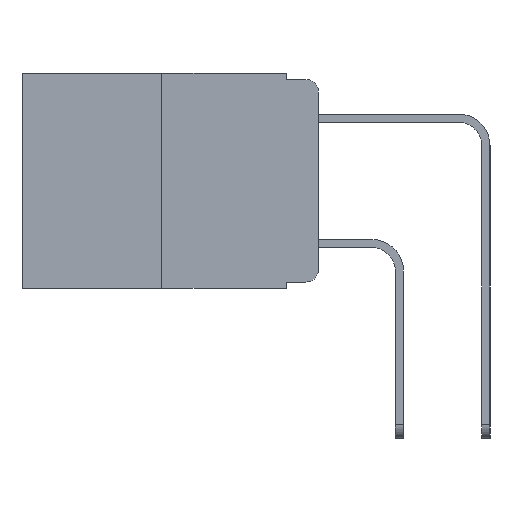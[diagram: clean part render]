
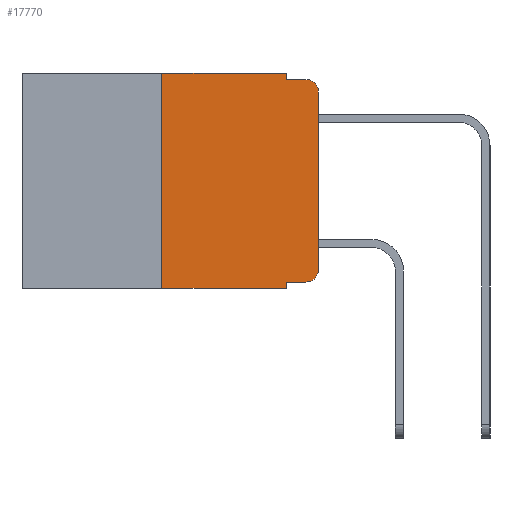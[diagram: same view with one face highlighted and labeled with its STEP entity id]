
A CAD part, left-side view. The second image highlights one B-rep face of the part: STEP entity #17770.
In plain terms, the highlighted planar face has unit normal (-1, 0, 0).
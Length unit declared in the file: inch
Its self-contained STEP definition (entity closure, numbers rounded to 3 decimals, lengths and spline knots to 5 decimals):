
#58 = VECTOR ( 'NONE', #22127, 39.37008 ) ;
#187 = DIRECTION ( 'NONE',  ( 0., 0., -1. ) ) ;
#230 = VERTEX_POINT ( 'NONE', #7218 ) ;
#246 = VERTEX_POINT ( 'NONE', #20464 ) ;
#477 = DIRECTION ( 'NONE',  ( 0., -1., 0. ) ) ;
#1325 = ORIENTED_EDGE ( 'NONE', *, *, #17352, .T. ) ;
#2344 = VERTEX_POINT ( 'NONE', #15406 ) ;
#2471 = VECTOR ( 'NONE', #20257, 39.37008 ) ;
#2782 = EDGE_LOOP ( 'NONE', ( #2958, #1325, #15148, #18935, #14340, #17602, #11539, #19645, #6774, #20719 ) ) ;
#2958 = ORIENTED_EDGE ( 'NONE', *, *, #18507, .T. ) ;
#3622 = CARTESIAN_POINT ( 'NONE',  ( 0., 0.25, 0. ) ) ;
#4239 = VERTEX_POINT ( 'NONE', #12228 ) ;
#4862 = CARTESIAN_POINT ( 'NONE',  ( 0., 0.051, 0. ) ) ;
#4883 = CARTESIAN_POINT ( 'NONE',  ( 0., 0.473, 0. ) ) ;
#5022 = LINE ( 'NONE', #14661, #21909 ) ;
#5245 = VERTEX_POINT ( 'NONE', #15235 ) ;
#5593 = EDGE_CURVE ( 'NONE', #4239, #2344, #10054, .T. ) ;
#6008 = VERTEX_POINT ( 'NONE', #19014 ) ;
#6492 = CARTESIAN_POINT ( 'NONE',  ( 0., 0.473, 0. ) ) ;
#6739 = EDGE_CURVE ( 'NONE', #15500, #4239, #17334, .T. ) ;
#6774 = ORIENTED_EDGE ( 'NONE', *, *, #6739, .T. ) ;
#6860 = DIRECTION ( 'NONE',  ( 0., 0., 1. ) ) ;
#7129 = VECTOR ( 'NONE', #15211, 39.37008 ) ;
#7173 = LINE ( 'NONE', #18534, #2471 ) ;
#7218 = CARTESIAN_POINT ( 'NONE',  ( 0., 0.051, 0. ) ) ;
#7348 = CARTESIAN_POINT ( 'NONE',  ( 0., 0.051, -0.333 ) ) ;
#7544 = VERTEX_POINT ( 'NONE', #15743 ) ;
#7870 = VERTEX_POINT ( 'NONE', #22075 ) ;
#7942 = EDGE_CURVE ( 'NONE', #15500, #246, #19655, .T. ) ;
#8250 = CARTESIAN_POINT ( 'NONE',  ( 0., 0.051, -0.01 ) ) ;
#8308 = DIRECTION ( 'NONE',  ( 0., 0., -1. ) ) ;
#8342 = LINE ( 'NONE', #4883, #12502 ) ;
#8681 = FACE_OUTER_BOUND ( 'NONE', #2782, .T. ) ;
#9966 = CARTESIAN_POINT ( 'NONE',  ( 0., 0.25, 0. ) ) ;
#10054 = CIRCLE ( 'NONE', #14104, 0.02 ) ;
#10192 = CARTESIAN_POINT ( 'NONE',  ( 0., 0.02, -0.03 ) ) ;
#10916 = DIRECTION ( 'NONE',  ( -1., 0., 0. ) ) ;
#10975 = EDGE_CURVE ( 'NONE', #19378, #230, #8342, .T. ) ;
#11064 = AXIS2_PLACEMENT_3D ( 'NONE', #10192, #22220, #11925 ) ;
#11522 = VECTOR ( 'NONE', #18910, 39.37008 ) ;
#11539 = ORIENTED_EDGE ( 'NONE', *, *, #13149, .T. ) ;
#11730 = VECTOR ( 'NONE', #6860, 39.37008 ) ;
#11866 = LINE ( 'NONE', #9966, #7129 ) ;
#11925 = DIRECTION ( 'NONE',  ( 0., 0., -1. ) ) ;
#12228 = CARTESIAN_POINT ( 'NONE',  ( 0., 0.02, -0.333 ) ) ;
#12502 = VECTOR ( 'NONE', #18928, 39.37008 ) ;
#12717 = EDGE_CURVE ( 'NONE', #7544, #19378, #11866, .T. ) ;
#12735 = VECTOR ( 'NONE', #22641, 39.37008 ) ;
#13149 = EDGE_CURVE ( 'NONE', #7544, #246, #5022, .T. ) ;
#13393 = CIRCLE ( 'NONE', #11064, 0.02 ) ;
#13555 = PLANE ( 'NONE',  #17605 ) ;
#13890 = EDGE_CURVE ( 'NONE', #230, #6008, #7173, .T. ) ;
#14104 = AXIS2_PLACEMENT_3D ( 'NONE', #21225, #10916, #187 ) ;
#14340 = ORIENTED_EDGE ( 'NONE', *, *, #10975, .F. ) ;
#14661 = CARTESIAN_POINT ( 'NONE',  ( 0., 0.473, -0.343 ) ) ;
#15148 = ORIENTED_EDGE ( 'NONE', *, *, #16191, .F. ) ;
#15211 = DIRECTION ( 'NONE',  ( 0., 0., 1. ) ) ;
#15235 = CARTESIAN_POINT ( 'NONE',  ( 0., 0., -0.03 ) ) ;
#15406 = CARTESIAN_POINT ( 'NONE',  ( 0., 0., -0.313 ) ) ;
#15500 = VERTEX_POINT ( 'NONE', #7348 ) ;
#15743 = CARTESIAN_POINT ( 'NONE',  ( 0., 0.25, -0.343 ) ) ;
#16191 = EDGE_CURVE ( 'NONE', #6008, #7870, #18868, .T. ) ;
#16339 = LINE ( 'NONE', #19130, #11730 ) ;
#17334 = LINE ( 'NONE', #19271, #12735 ) ;
#17352 = EDGE_CURVE ( 'NONE', #5245, #7870, #13393, .T. ) ;
#17602 = ORIENTED_EDGE ( 'NONE', *, *, #12717, .F. ) ;
#17605 = AXIS2_PLACEMENT_3D ( 'NONE', #6492, #18771, #8308 ) ;
#17770 = ADVANCED_FACE ( 'NONE', ( #8681 ), #13555, .F. ) ;
#18507 = EDGE_CURVE ( 'NONE', #2344, #5245, #16339, .T. ) ;
#18534 = CARTESIAN_POINT ( 'NONE',  ( 0., 0.051, 0. ) ) ;
#18771 = DIRECTION ( 'NONE',  ( 1., 0., 0. ) ) ;
#18868 = LINE ( 'NONE', #8250, #58 ) ;
#18910 = DIRECTION ( 'NONE',  ( 0., 0., -1. ) ) ;
#18928 = DIRECTION ( 'NONE',  ( 0., -1., 0. ) ) ;
#18935 = ORIENTED_EDGE ( 'NONE', *, *, #13890, .F. ) ;
#19014 = CARTESIAN_POINT ( 'NONE',  ( 0., 0.051, -0.01 ) ) ;
#19130 = CARTESIAN_POINT ( 'NONE',  ( 0., 0., 0. ) ) ;
#19271 = CARTESIAN_POINT ( 'NONE',  ( 0., 0.051, -0.333 ) ) ;
#19378 = VERTEX_POINT ( 'NONE', #3622 ) ;
#19645 = ORIENTED_EDGE ( 'NONE', *, *, #7942, .F. ) ;
#19655 = LINE ( 'NONE', #4862, #11522 ) ;
#20257 = DIRECTION ( 'NONE',  ( 0., 0., -1. ) ) ;
#20464 = CARTESIAN_POINT ( 'NONE',  ( 0., 0.051, -0.343 ) ) ;
#20719 = ORIENTED_EDGE ( 'NONE', *, *, #5593, .T. ) ;
#21225 = CARTESIAN_POINT ( 'NONE',  ( 0., 0.02, -0.313 ) ) ;
#21909 = VECTOR ( 'NONE', #477, 39.37008 ) ;
#22075 = CARTESIAN_POINT ( 'NONE',  ( 0., 0.02, -0.01 ) ) ;
#22127 = DIRECTION ( 'NONE',  ( 0., -1., 0. ) ) ;
#22220 = DIRECTION ( 'NONE',  ( -1., 0., 0. ) ) ;
#22641 = DIRECTION ( 'NONE',  ( 0., -1., 0. ) ) ;
